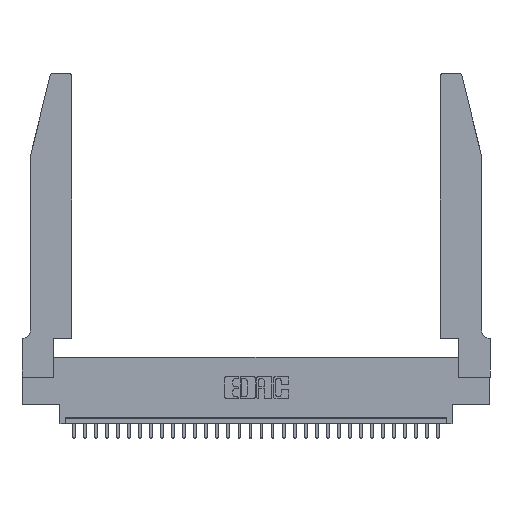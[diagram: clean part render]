
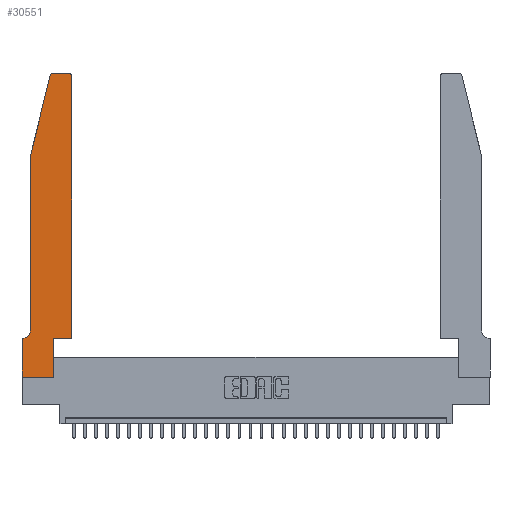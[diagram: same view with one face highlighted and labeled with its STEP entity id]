
A CAD part, top view. The second image highlights one B-rep face of the part: STEP entity #30551.
In plain terms, the highlighted planar face has unit normal (0, 0, 1).
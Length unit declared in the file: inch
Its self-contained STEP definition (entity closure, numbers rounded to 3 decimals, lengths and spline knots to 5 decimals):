
#478 = CARTESIAN_POINT ( 'NONE',  ( 0.4205, 2.75, 0.37 ) ) ;
#558 = EDGE_CURVE ( 'NONE', #30779, #30566, #25909, .T. ) ;
#873 = CARTESIAN_POINT ( 'NONE',  ( 0.284, 2.72, 0.37 ) ) ;
#1079 = DIRECTION ( 'NONE',  ( 0., -1., 0. ) ) ;
#1468 = VERTEX_POINT ( 'NONE', #20734 ) ;
#1542 = EDGE_CURVE ( 'NONE', #15246, #16303, #21646, .T. ) ;
#1728 = CARTESIAN_POINT ( 'NONE',  ( 0.2605, 2.75, 0.37 ) ) ;
#1777 = ORIENTED_EDGE ( 'NONE', *, *, #27989, .T. ) ;
#2006 = CARTESIAN_POINT ( 'NONE',  ( 0., 0.35, 0.37 ) ) ;
#2492 = EDGE_LOOP ( 'NONE', ( #22299, #19825, #24276, #1777, #18628, #4856, #14361, #7342, #14746, #18948, #6942, #9615 ) ) ;
#3371 = DIRECTION ( 'NONE',  ( 0., 1., 0. ) ) ;
#3542 = LINE ( 'NONE', #30901, #12644 ) ;
#3680 = CIRCLE ( 'NONE', #28759, 0.07 ) ;
#3739 = LINE ( 'NONE', #20451, #10937 ) ;
#3799 = EDGE_CURVE ( 'NONE', #17197, #30779, #28382, .T. ) ;
#4335 = DIRECTION ( 'NONE',  ( 0., 0., 1. ) ) ;
#4655 = PLANE ( 'NONE',  #30331 ) ;
#4834 = CARTESIAN_POINT ( 'NONE',  ( 0.4505, 0.35, 0.37 ) ) ;
#4856 = ORIENTED_EDGE ( 'NONE', *, *, #28486, .T. ) ;
#4910 = EDGE_CURVE ( 'NONE', #17135, #15246, #3542, .T. ) ;
#5123 = CARTESIAN_POINT ( 'NONE',  ( 0.0055, 0.42, 0.37 ) ) ;
#5888 = AXIS2_PLACEMENT_3D ( 'NONE', #21483, #6859, #21594 ) ;
#6370 = DIRECTION ( 'NONE',  ( -0.239, -0.971, 0. ) ) ;
#6859 = DIRECTION ( 'NONE',  ( 0., 0., 1. ) ) ;
#6942 = ORIENTED_EDGE ( 'NONE', *, *, #4910, .T. ) ;
#6987 = VECTOR ( 'NONE', #9381, 39.37008 ) ;
#7342 = ORIENTED_EDGE ( 'NONE', *, *, #558, .T. ) ;
#7775 = DIRECTION ( 'NONE',  ( -1., 0., 0. ) ) ;
#8168 = CARTESIAN_POINT ( 'NONE',  ( 0.0755, 2., 0.37 ) ) ;
#8184 = DIRECTION ( 'NONE',  ( 0., 0., 1. ) ) ;
#8577 = CARTESIAN_POINT ( 'NONE',  ( 0.25487, 2.72718, 0.37 ) ) ;
#9113 = CARTESIAN_POINT ( 'NONE',  ( 0.2865, 0., 0.37 ) ) ;
#9381 = DIRECTION ( 'NONE',  ( 1., 0., 0. ) ) ;
#9615 = ORIENTED_EDGE ( 'NONE', *, *, #1542, .T. ) ;
#10777 = CARTESIAN_POINT ( 'NONE',  ( 0.4505, 2.72, 0.37 ) ) ;
#10831 = LINE ( 'NONE', #20989, #22365 ) ;
#10937 = VECTOR ( 'NONE', #27655, 39.37008 ) ;
#11287 = DIRECTION ( 'NONE',  ( 1., 0., 0. ) ) ;
#12045 = VECTOR ( 'NONE', #18873, 39.37008 ) ;
#12500 = LINE ( 'NONE', #20486, #30099 ) ;
#12574 = EDGE_CURVE ( 'NONE', #15102, #20997, #3680, .T. ) ;
#12644 = VECTOR ( 'NONE', #20911, 39.37008 ) ;
#14361 = ORIENTED_EDGE ( 'NONE', *, *, #3799, .T. ) ;
#14746 = ORIENTED_EDGE ( 'NONE', *, *, #18087, .T. ) ;
#15102 = VERTEX_POINT ( 'NONE', #24849 ) ;
#15246 = VERTEX_POINT ( 'NONE', #10777 ) ;
#16303 = VERTEX_POINT ( 'NONE', #478 ) ;
#16989 = VERTEX_POINT ( 'NONE', #8168 ) ;
#17135 = VERTEX_POINT ( 'NONE', #28195 ) ;
#17141 = EDGE_CURVE ( 'NONE', #24874, #16989, #10831, .T. ) ;
#17197 = VERTEX_POINT ( 'NONE', #30762 ) ;
#18007 = DIRECTION ( 'NONE',  ( 1., 0., 0. ) ) ;
#18087 = EDGE_CURVE ( 'NONE', #30566, #1468, #27954, .T. ) ;
#18168 = LINE ( 'NONE', #1728, #12045 ) ;
#18628 = ORIENTED_EDGE ( 'NONE', *, *, #12574, .T. ) ;
#18873 = DIRECTION ( 'NONE',  ( -1., 0., 0. ) ) ;
#18948 = ORIENTED_EDGE ( 'NONE', *, *, #31197, .T. ) ;
#19112 = CARTESIAN_POINT ( 'NONE',  ( 0.0055, 0.35, 0.37 ) ) ;
#19254 = FACE_OUTER_BOUND ( 'NONE', #2492, .T. ) ;
#19630 = DIRECTION ( 'NONE',  ( 0., 0., -1. ) ) ;
#19825 = ORIENTED_EDGE ( 'NONE', *, *, #24410, .T. ) ;
#20417 = VECTOR ( 'NONE', #23791, 39.37008 ) ;
#20451 = CARTESIAN_POINT ( 'NONE',  ( 0.0755, 0.35, 0.37 ) ) ;
#20486 = CARTESIAN_POINT ( 'NONE',  ( 0.0755, 2., 0.37 ) ) ;
#20734 = CARTESIAN_POINT ( 'NONE',  ( 0.2865, 0.35, 0.37 ) ) ;
#20911 = DIRECTION ( 'NONE',  ( 0., 1., 0. ) ) ;
#20989 = CARTESIAN_POINT ( 'NONE',  ( 0.0755, 2., 0.37 ) ) ;
#20997 = VERTEX_POINT ( 'NONE', #19112 ) ;
#21416 = DIRECTION ( 'NONE',  ( 1., 0., 0. ) ) ;
#21483 = CARTESIAN_POINT ( 'NONE',  ( 0.4205, 2.72, 0.37 ) ) ;
#21594 = DIRECTION ( 'NONE',  ( 1., 0., 0. ) ) ;
#21646 = CIRCLE ( 'NONE', #5888, 0.03 ) ;
#22299 = ORIENTED_EDGE ( 'NONE', *, *, #23409, .T. ) ;
#22340 = CIRCLE ( 'NONE', #24968, 0.03 ) ;
#22365 = VECTOR ( 'NONE', #6370, 39.37008 ) ;
#23409 = EDGE_CURVE ( 'NONE', #16303, #29467, #18168, .T. ) ;
#23691 = CARTESIAN_POINT ( 'NONE',  ( 0., 0., 0.37 ) ) ;
#23791 = DIRECTION ( 'NONE',  ( 0., -1., 0. ) ) ;
#23922 = CARTESIAN_POINT ( 'NONE',  ( 0., 0., 0.37 ) ) ;
#24276 = ORIENTED_EDGE ( 'NONE', *, *, #17141, .T. ) ;
#24410 = EDGE_CURVE ( 'NONE', #29467, #24874, #22340, .T. ) ;
#24776 = VECTOR ( 'NONE', #11287, 39.37008 ) ;
#24849 = CARTESIAN_POINT ( 'NONE',  ( 0.0755, 0.42, 0.37 ) ) ;
#24874 = VERTEX_POINT ( 'NONE', #8577 ) ;
#24968 = AXIS2_PLACEMENT_3D ( 'NONE', #873, #8184, #18007 ) ;
#25909 = LINE ( 'NONE', #23922, #24776 ) ;
#27205 = CARTESIAN_POINT ( 'NONE',  ( 0.284, 2.75, 0.37 ) ) ;
#27650 = CARTESIAN_POINT ( 'NONE',  ( 0.2865, 0.35, 0.37 ) ) ;
#27655 = DIRECTION ( 'NONE',  ( -1., 0., 0. ) ) ;
#27940 = LINE ( 'NONE', #4834, #6987 ) ;
#27954 = LINE ( 'NONE', #27650, #28734 ) ;
#27989 = EDGE_CURVE ( 'NONE', #16989, #15102, #12500, .T. ) ;
#28195 = CARTESIAN_POINT ( 'NONE',  ( 0.4505, 0.35, 0.37 ) ) ;
#28382 = LINE ( 'NONE', #23691, #20417 ) ;
#28486 = EDGE_CURVE ( 'NONE', #20997, #17197, #3739, .T. ) ;
#28734 = VECTOR ( 'NONE', #3371, 39.37008 ) ;
#28759 = AXIS2_PLACEMENT_3D ( 'NONE', #5123, #19630, #7775 ) ;
#29144 = CARTESIAN_POINT ( 'NONE',  ( 0., 0., 0.37 ) ) ;
#29467 = VERTEX_POINT ( 'NONE', #27205 ) ;
#30099 = VECTOR ( 'NONE', #1079, 39.37008 ) ;
#30331 = AXIS2_PLACEMENT_3D ( 'NONE', #2006, #4335, #21416 ) ;
#30551 = ADVANCED_FACE ( 'NONE', ( #19254 ), #4655, .T. ) ;
#30566 = VERTEX_POINT ( 'NONE', #9113 ) ;
#30762 = CARTESIAN_POINT ( 'NONE',  ( 0., 0.35, 0.37 ) ) ;
#30779 = VERTEX_POINT ( 'NONE', #29144 ) ;
#30901 = CARTESIAN_POINT ( 'NONE',  ( 0.4505, 0.35, 0.37 ) ) ;
#31197 = EDGE_CURVE ( 'NONE', #1468, #17135, #27940, .T. ) ;
